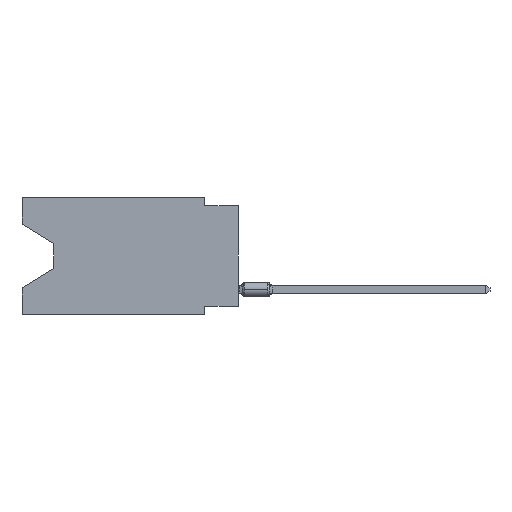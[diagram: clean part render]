
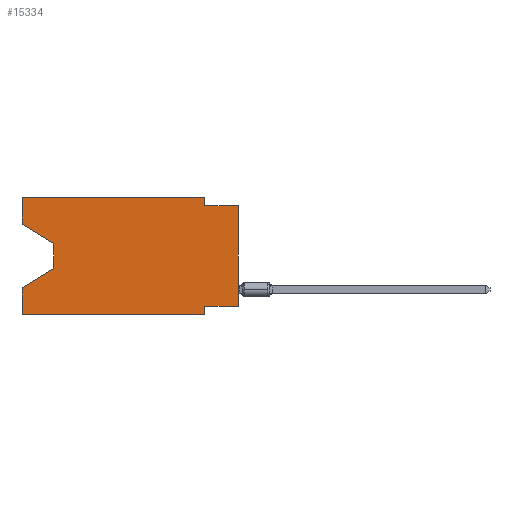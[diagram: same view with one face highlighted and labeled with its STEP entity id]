
A CAD part, left-side view. The second image highlights one B-rep face of the part: STEP entity #15334.
In plain terms, the highlighted planar face has unit normal (-1, 0, 0).
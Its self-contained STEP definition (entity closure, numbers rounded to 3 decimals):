
#243 = CARTESIAN_POINT ( 'NONE',  ( 0., 16.383, 0. ) ) ;
#816 = ORIENTED_EDGE ( 'NONE', *, *, #9080, .F. ) ;
#949 = VECTOR ( 'NONE', #15721, 1000. ) ;
#950 = CARTESIAN_POINT ( 'NONE',  ( 0., 16.383, -6.852 ) ) ;
#1576 = CARTESIAN_POINT ( 'NONE',  ( 0., 16.383, -8.89 ) ) ;
#1801 = CARTESIAN_POINT ( 'NONE',  ( 0., 16.383, 0. ) ) ;
#1981 = CARTESIAN_POINT ( 'NONE',  ( 0., 13.97, -3.505 ) ) ;
#2014 = CARTESIAN_POINT ( 'NONE',  ( 0., 0., -0.635 ) ) ;
#2083 = VECTOR ( 'NONE', #10252, 1000. ) ;
#2087 = LINE ( 'NONE', #5663, #22889 ) ;
#2447 = VERTEX_POINT ( 'NONE', #950 ) ;
#2452 = CARTESIAN_POINT ( 'NONE',  ( 0., 16.383, 0. ) ) ;
#2604 = ORIENTED_EDGE ( 'NONE', *, *, #22503, .F. ) ;
#2786 = ORIENTED_EDGE ( 'NONE', *, *, #19227, .F. ) ;
#3393 = EDGE_CURVE ( 'NONE', #12686, #14044, #5008, .T. ) ;
#3651 = DIRECTION ( 'NONE',  ( 0., -1., 0. ) ) ;
#4098 = VECTOR ( 'NONE', #11557, 1000. ) ;
#4176 = DIRECTION ( 'NONE',  ( 0., 0., -1. ) ) ;
#4300 = LINE ( 'NONE', #2452, #20213 ) ;
#4667 = CARTESIAN_POINT ( 'NONE',  ( 0., 16.383, -2.038 ) ) ;
#4729 = CARTESIAN_POINT ( 'NONE',  ( 0., 16.383, 0. ) ) ;
#4744 = EDGE_CURVE ( 'NONE', #18136, #5095, #6390, .T. ) ;
#5008 = LINE ( 'NONE', #14336, #9208 ) ;
#5095 = VERTEX_POINT ( 'NONE', #22621 ) ;
#5243 = CARTESIAN_POINT ( 'NONE',  ( 0., 2.54, -8.255 ) ) ;
#5513 = LINE ( 'NONE', #9448, #23821 ) ;
#5663 = CARTESIAN_POINT ( 'NONE',  ( 0., 2.54, -8.89 ) ) ;
#5946 = ORIENTED_EDGE ( 'NONE', *, *, #14582, .T. ) ;
#6307 = ORIENTED_EDGE ( 'NONE', *, *, #23782, .T. ) ;
#6390 = LINE ( 'NONE', #4667, #13561 ) ;
#6460 = CARTESIAN_POINT ( 'NONE',  ( 0., 0., -8.255 ) ) ;
#7219 = VECTOR ( 'NONE', #23656, 1000. ) ;
#7591 = DIRECTION ( 'NONE',  ( 0., -1., 0. ) ) ;
#7616 = DIRECTION ( 'NONE',  ( 1., 0., 0. ) ) ;
#7722 = VECTOR ( 'NONE', #19366, 1000. ) ;
#7745 = VERTEX_POINT ( 'NONE', #23150 ) ;
#7756 = LINE ( 'NONE', #20912, #949 ) ;
#8540 = CARTESIAN_POINT ( 'NONE',  ( 0., 16.383, -8.89 ) ) ;
#8656 = LINE ( 'NONE', #8540, #7219 ) ;
#9080 = EDGE_CURVE ( 'NONE', #14044, #16469, #5513, .T. ) ;
#9182 = CARTESIAN_POINT ( 'NONE',  ( 0., 16.383, -2.038 ) ) ;
#9208 = VECTOR ( 'NONE', #3651, 1000. ) ;
#9346 = FACE_OUTER_BOUND ( 'NONE', #11443, .T. ) ;
#9448 = CARTESIAN_POINT ( 'NONE',  ( 0., 2.54, 0. ) ) ;
#9799 = LINE ( 'NONE', #11762, #17086 ) ;
#10252 = DIRECTION ( 'NONE',  ( 0., 1., 0. ) ) ;
#11443 = EDGE_LOOP ( 'NONE', ( #17900, #5946, #18852, #23977, #6307, #15534, #2604, #13061, #2786, #816, #21595, #23634 ) ) ;
#11557 = DIRECTION ( 'NONE',  ( 0., 0., -1. ) ) ;
#11762 = CARTESIAN_POINT ( 'NONE',  ( 0., 0., -0.635 ) ) ;
#12032 = EDGE_CURVE ( 'NONE', #12945, #2447, #4300, .T. ) ;
#12223 = LINE ( 'NONE', #4729, #7722 ) ;
#12236 = CARTESIAN_POINT ( 'NONE',  ( 0., 2.54, 0. ) ) ;
#12319 = CARTESIAN_POINT ( 'NONE',  ( 0., 2.54, -0.635 ) ) ;
#12685 = VECTOR ( 'NONE', #14859, 1000. ) ;
#12686 = VERTEX_POINT ( 'NONE', #1801 ) ;
#12945 = VERTEX_POINT ( 'NONE', #1576 ) ;
#13061 = ORIENTED_EDGE ( 'NONE', *, *, #23078, .T. ) ;
#13067 = CARTESIAN_POINT ( 'NONE',  ( 0., 13.97, -5.385 ) ) ;
#13458 = EDGE_CURVE ( 'NONE', #15653, #7745, #2087, .T. ) ;
#13561 = VECTOR ( 'NONE', #15726, 1000. ) ;
#14044 = VERTEX_POINT ( 'NONE', #12236 ) ;
#14108 = DIRECTION ( 'NONE',  ( 0., 0., 1. ) ) ;
#14156 = CARTESIAN_POINT ( 'NONE',  ( 0., 0., -8.255 ) ) ;
#14336 = CARTESIAN_POINT ( 'NONE',  ( 0., 16.383, 0. ) ) ;
#14582 = EDGE_CURVE ( 'NONE', #5095, #21168, #18946, .T. ) ;
#14639 = EDGE_CURVE ( 'NONE', #21168, #2447, #7756, .T. ) ;
#14859 = DIRECTION ( 'NONE',  ( 0., 0., 1. ) ) ;
#15334 = ADVANCED_FACE ( 'NONE', ( #9346 ), #22857, .F. ) ;
#15534 = ORIENTED_EDGE ( 'NONE', *, *, #13458, .F. ) ;
#15653 = VERTEX_POINT ( 'NONE', #5243 ) ;
#15721 = DIRECTION ( 'NONE',  ( 0., 0.855, -0.519 ) ) ;
#15726 = DIRECTION ( 'NONE',  ( 0., -0.855, -0.519 ) ) ;
#16459 = VERTEX_POINT ( 'NONE', #14156 ) ;
#16469 = VERTEX_POINT ( 'NONE', #12319 ) ;
#16711 = CARTESIAN_POINT ( 'NONE',  ( 0., 0., 0. ) ) ;
#16938 = DIRECTION ( 'NONE',  ( 0., 0., -1. ) ) ;
#17075 = AXIS2_PLACEMENT_3D ( 'NONE', #243, #7616, #4176 ) ;
#17086 = VECTOR ( 'NONE', #7591, 1000. ) ;
#17290 = EDGE_CURVE ( 'NONE', #18136, #12686, #12223, .T. ) ;
#17900 = ORIENTED_EDGE ( 'NONE', *, *, #4744, .T. ) ;
#18136 = VERTEX_POINT ( 'NONE', #9182 ) ;
#18852 = ORIENTED_EDGE ( 'NONE', *, *, #14639, .T. ) ;
#18946 = LINE ( 'NONE', #1981, #4098 ) ;
#19227 = EDGE_CURVE ( 'NONE', #16469, #21171, #9799, .T. ) ;
#19366 = DIRECTION ( 'NONE',  ( 0., 0., 1. ) ) ;
#20213 = VECTOR ( 'NONE', #14108, 1000. ) ;
#20912 = CARTESIAN_POINT ( 'NONE',  ( 0., 13.97, -5.385 ) ) ;
#21168 = VERTEX_POINT ( 'NONE', #13067 ) ;
#21171 = VERTEX_POINT ( 'NONE', #2014 ) ;
#21595 = ORIENTED_EDGE ( 'NONE', *, *, #3393, .F. ) ;
#22503 = EDGE_CURVE ( 'NONE', #16459, #15653, #23295, .T. ) ;
#22621 = CARTESIAN_POINT ( 'NONE',  ( 0., 13.97, -3.505 ) ) ;
#22857 = PLANE ( 'NONE',  #17075 ) ;
#22889 = VECTOR ( 'NONE', #24237, 1000. ) ;
#23078 = EDGE_CURVE ( 'NONE', #16459, #21171, #23624, .T. ) ;
#23150 = CARTESIAN_POINT ( 'NONE',  ( 0., 2.54, -8.89 ) ) ;
#23295 = LINE ( 'NONE', #6460, #2083 ) ;
#23624 = LINE ( 'NONE', #16711, #12685 ) ;
#23634 = ORIENTED_EDGE ( 'NONE', *, *, #17290, .F. ) ;
#23656 = DIRECTION ( 'NONE',  ( 0., -1., 0. ) ) ;
#23782 = EDGE_CURVE ( 'NONE', #12945, #7745, #8656, .T. ) ;
#23821 = VECTOR ( 'NONE', #16938, 1000. ) ;
#23977 = ORIENTED_EDGE ( 'NONE', *, *, #12032, .F. ) ;
#24237 = DIRECTION ( 'NONE',  ( 0., 0., -1. ) ) ;
